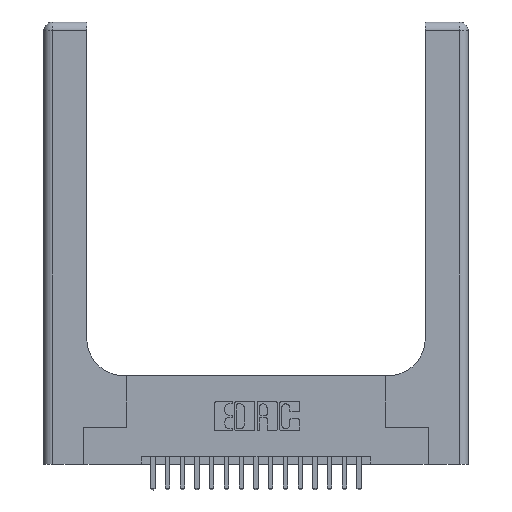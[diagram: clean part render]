
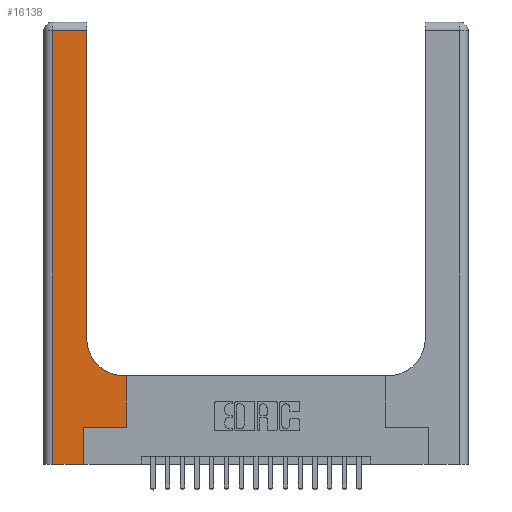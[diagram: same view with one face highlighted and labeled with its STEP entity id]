
A CAD part, top view. The second image highlights one B-rep face of the part: STEP entity #16138.
In plain terms, the highlighted planar face has unit normal (0, 0, 1).
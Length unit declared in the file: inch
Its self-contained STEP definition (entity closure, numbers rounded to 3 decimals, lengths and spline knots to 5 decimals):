
#85 = VERTEX_POINT ( 'NONE', #20459 ) ;
#296 = VERTEX_POINT ( 'NONE', #11127 ) ;
#655 = DIRECTION ( 'NONE',  ( 0., 1., 0. ) ) ;
#1073 = LINE ( 'NONE', #1368, #10759 ) ;
#1085 = LINE ( 'NONE', #13766, #17862 ) ;
#1368 = CARTESIAN_POINT ( 'NONE',  ( 0.269, 0., 0.37 ) ) ;
#1416 = VECTOR ( 'NONE', #12512, 39.37008 ) ;
#2290 = AXIS2_PLACEMENT_3D ( 'NONE', #7629, #17179, #6183 ) ;
#2315 = LINE ( 'NONE', #9566, #12778 ) ;
#3492 = CARTESIAN_POINT ( 'NONE',  ( 0.269, 0.25, 0.37 ) ) ;
#3637 = VERTEX_POINT ( 'NONE', #8293 ) ;
#3656 = EDGE_LOOP ( 'NONE', ( #19562, #19521, #18984, #20089, #8980, #6480, #10608, #17317, #9600 ) ) ;
#3802 = DIRECTION ( 'NONE',  ( 0., 0., -1. ) ) ;
#4604 = VERTEX_POINT ( 'NONE', #3492 ) ;
#5599 = LINE ( 'NONE', #16175, #16889 ) ;
#6183 = DIRECTION ( 'NONE',  ( -1., 0., 0. ) ) ;
#6480 = ORIENTED_EDGE ( 'NONE', *, *, #16304, .T. ) ;
#7182 = EDGE_CURVE ( 'NONE', #13927, #15580, #16754, .T. ) ;
#7316 = CARTESIAN_POINT ( 'NONE',  ( 0.5585, 0.25, 0.37 ) ) ;
#7473 = CARTESIAN_POINT ( 'NONE',  ( 0.2915, 0.85, 0.37 ) ) ;
#7629 = CARTESIAN_POINT ( 'NONE',  ( 0., 3., 0.37 ) ) ;
#7706 = VERTEX_POINT ( 'NONE', #7316 ) ;
#8293 = CARTESIAN_POINT ( 'NONE',  ( 0.06, 2.94, 0.37 ) ) ;
#8722 = CARTESIAN_POINT ( 'NONE',  ( 0.5585, 0.25, 0.37 ) ) ;
#8980 = ORIENTED_EDGE ( 'NONE', *, *, #16142, .T. ) ;
#9140 = VERTEX_POINT ( 'NONE', #14045 ) ;
#9204 = LINE ( 'NONE', #19102, #17790 ) ;
#9292 = DIRECTION ( 'NONE',  ( 0., 1., 0. ) ) ;
#9566 = CARTESIAN_POINT ( 'NONE',  ( 0.269, 0.25, 0.37 ) ) ;
#9600 = ORIENTED_EDGE ( 'NONE', *, *, #16427, .T. ) ;
#9765 = DIRECTION ( 'NONE',  ( 1., 0., 0. ) ) ;
#9919 = DIRECTION ( 'NONE',  ( 1., 0., 0. ) ) ;
#10608 = ORIENTED_EDGE ( 'NONE', *, *, #12043, .T. ) ;
#10759 = VECTOR ( 'NONE', #9292, 39.37008 ) ;
#11127 = CARTESIAN_POINT ( 'NONE',  ( 0.5585, 0.6, 0.37 ) ) ;
#11503 = EDGE_CURVE ( 'NONE', #3637, #19675, #1085, .T. ) ;
#12043 = EDGE_CURVE ( 'NONE', #7706, #296, #18826, .T. ) ;
#12214 = DIRECTION ( 'NONE',  ( 0., -1., 0. ) ) ;
#12460 = VECTOR ( 'NONE', #13989, 39.37008 ) ;
#12512 = DIRECTION ( 'NONE',  ( -1., 0., 0. ) ) ;
#12536 = FACE_OUTER_BOUND ( 'NONE', #3656, .T. ) ;
#12778 = VECTOR ( 'NONE', #9765, 39.37008 ) ;
#12794 = VECTOR ( 'NONE', #655, 39.37008 ) ;
#13766 = CARTESIAN_POINT ( 'NONE',  ( 0.06, 3., 0.37 ) ) ;
#13927 = VERTEX_POINT ( 'NONE', #7473 ) ;
#13989 = DIRECTION ( 'NONE',  ( 0., 1., 0. ) ) ;
#14045 = CARTESIAN_POINT ( 'NONE',  ( 0.269, 0., 0.37 ) ) ;
#14316 = DIRECTION ( 'NONE',  ( -1., 0., 0. ) ) ;
#14667 = LINE ( 'NONE', #20491, #1416 ) ;
#14787 = EDGE_CURVE ( 'NONE', #19675, #9140, #5599, .T. ) ;
#15580 = VERTEX_POINT ( 'NONE', #16058 ) ;
#15609 = CARTESIAN_POINT ( 'NONE',  ( 0.2915, 3., 0.37 ) ) ;
#16044 = CIRCLE ( 'NONE', #17176, 0.25 ) ;
#16058 = CARTESIAN_POINT ( 'NONE',  ( 0.2915, 2.94, 0.37 ) ) ;
#16138 = ADVANCED_FACE ( 'NONE', ( #12536 ), #17324, .F. ) ;
#16142 = EDGE_CURVE ( 'NONE', #9140, #4604, #1073, .T. ) ;
#16175 = CARTESIAN_POINT ( 'NONE',  ( 0., 0., 0.37 ) ) ;
#16304 = EDGE_CURVE ( 'NONE', #4604, #7706, #2315, .T. ) ;
#16427 = EDGE_CURVE ( 'NONE', #85, #13927, #16044, .T. ) ;
#16754 = LINE ( 'NONE', #15609, #12460 ) ;
#16889 = VECTOR ( 'NONE', #9919, 39.37008 ) ;
#17176 = AXIS2_PLACEMENT_3D ( 'NONE', #17891, #3802, #19597 ) ;
#17179 = DIRECTION ( 'NONE',  ( 0., 0., -1. ) ) ;
#17317 = ORIENTED_EDGE ( 'NONE', *, *, #18320, .T. ) ;
#17324 = PLANE ( 'NONE',  #2290 ) ;
#17790 = VECTOR ( 'NONE', #14316, 39.37008 ) ;
#17862 = VECTOR ( 'NONE', #12214, 39.37008 ) ;
#17891 = CARTESIAN_POINT ( 'NONE',  ( 0.5415, 0.85, 0.37 ) ) ;
#18290 = CARTESIAN_POINT ( 'NONE',  ( 0.06, 0., 0.37 ) ) ;
#18320 = EDGE_CURVE ( 'NONE', #296, #85, #9204, .T. ) ;
#18826 = LINE ( 'NONE', #8722, #12794 ) ;
#18984 = ORIENTED_EDGE ( 'NONE', *, *, #11503, .T. ) ;
#19102 = CARTESIAN_POINT ( 'NONE',  ( 0.2915, 0.6, 0.37 ) ) ;
#19521 = ORIENTED_EDGE ( 'NONE', *, *, #20290, .T. ) ;
#19562 = ORIENTED_EDGE ( 'NONE', *, *, #7182, .T. ) ;
#19597 = DIRECTION ( 'NONE',  ( 1., 0., 0. ) ) ;
#19675 = VERTEX_POINT ( 'NONE', #18290 ) ;
#20089 = ORIENTED_EDGE ( 'NONE', *, *, #14787, .T. ) ;
#20290 = EDGE_CURVE ( 'NONE', #15580, #3637, #14667, .T. ) ;
#20459 = CARTESIAN_POINT ( 'NONE',  ( 0.5415, 0.6, 0.37 ) ) ;
#20491 = CARTESIAN_POINT ( 'NONE',  ( 0., 2.94, 0.37 ) ) ;
